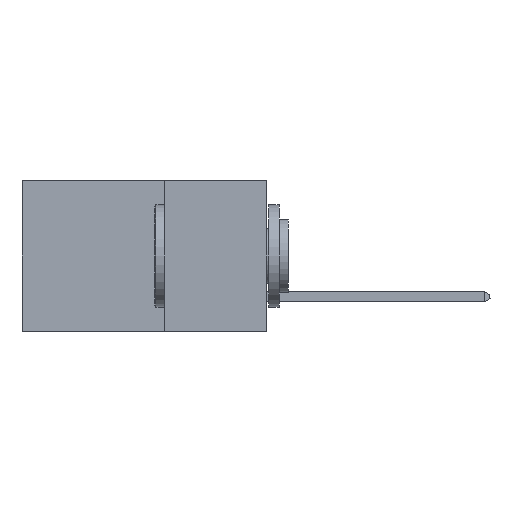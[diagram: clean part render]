
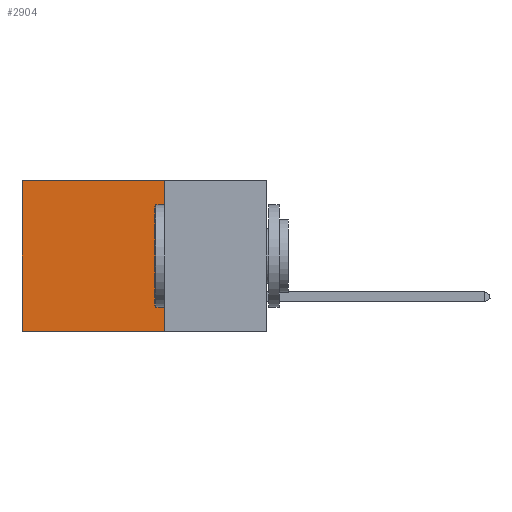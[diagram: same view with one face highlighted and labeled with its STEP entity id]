
A CAD part, left-side view. The second image highlights one B-rep face of the part: STEP entity #2904.
In plain terms, the highlighted planar face has unit normal (-1, 0, 0).
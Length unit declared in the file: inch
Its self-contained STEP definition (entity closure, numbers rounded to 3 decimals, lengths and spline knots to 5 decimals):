
#697 = CARTESIAN_POINT ( 'NONE',  ( 0.2875, 0.25, -0.37 ) ) ;
#1214 = VERTEX_POINT ( 'NONE', #697 ) ;
#2812 = DIRECTION ( 'NONE',  ( 0., 0., -1. ) ) ;
#2901 = CARTESIAN_POINT ( 'NONE',  ( 0.2875, 0.6, -0.37 ) ) ;
#2904 = ADVANCED_FACE ( 'NONE', ( #7168 ), #30668, .F. ) ;
#3519 = CARTESIAN_POINT ( 'NONE',  ( 0.2875, 0.25, 0. ) ) ;
#3806 = ORIENTED_EDGE ( 'NONE', *, *, #16122, .T. ) ;
#3827 = DIRECTION ( 'NONE',  ( 1., 0., 0. ) ) ;
#6493 = VECTOR ( 'NONE', #12857, 39.37008 ) ;
#7168 = FACE_OUTER_BOUND ( 'NONE', #11934, .T. ) ;
#8138 = ORIENTED_EDGE ( 'NONE', *, *, #24758, .F. ) ;
#8615 = VERTEX_POINT ( 'NONE', #20399 ) ;
#8788 = LINE ( 'NONE', #24919, #6493 ) ;
#8815 = VERTEX_POINT ( 'NONE', #28167 ) ;
#9678 = VERTEX_POINT ( 'NONE', #2901 ) ;
#10914 = DIRECTION ( 'NONE',  ( 0., 0., -1. ) ) ;
#11934 = EDGE_LOOP ( 'NONE', ( #28838, #25060, #8138, #3806 ) ) ;
#12069 = LINE ( 'NONE', #22989, #26578 ) ;
#12084 = EDGE_CURVE ( 'NONE', #8615, #9678, #18480, .T. ) ;
#12692 = VECTOR ( 'NONE', #2812, 39.37008 ) ;
#12857 = DIRECTION ( 'NONE',  ( 0., 1., 0. ) ) ;
#13100 = CARTESIAN_POINT ( 'NONE',  ( 0.2875, 0.25, -0.37 ) ) ;
#13912 = AXIS2_PLACEMENT_3D ( 'NONE', #3519, #3827, #10914 ) ;
#16122 = EDGE_CURVE ( 'NONE', #8815, #8615, #8788, .T. ) ;
#18480 = LINE ( 'NONE', #29619, #12692 ) ;
#20399 = CARTESIAN_POINT ( 'NONE',  ( 0.2875, 0.6, 0. ) ) ;
#20895 = EDGE_CURVE ( 'NONE', #1214, #9678, #28010, .T. ) ;
#22989 = CARTESIAN_POINT ( 'NONE',  ( 0.2875, 0.25, 0. ) ) ;
#24758 = EDGE_CURVE ( 'NONE', #8815, #1214, #12069, .T. ) ;
#24919 = CARTESIAN_POINT ( 'NONE',  ( 0.2875, 0.25, 0. ) ) ;
#25060 = ORIENTED_EDGE ( 'NONE', *, *, #20895, .F. ) ;
#25523 = DIRECTION ( 'NONE',  ( 0., 0., -1. ) ) ;
#26578 = VECTOR ( 'NONE', #25523, 39.37008 ) ;
#28010 = LINE ( 'NONE', #13100, #28772 ) ;
#28167 = CARTESIAN_POINT ( 'NONE',  ( 0.2875, 0.25, 0. ) ) ;
#28772 = VECTOR ( 'NONE', #30184, 39.37008 ) ;
#28838 = ORIENTED_EDGE ( 'NONE', *, *, #12084, .T. ) ;
#29619 = CARTESIAN_POINT ( 'NONE',  ( 0.2875, 0.6, 0. ) ) ;
#30184 = DIRECTION ( 'NONE',  ( 0., 1., 0. ) ) ;
#30668 = PLANE ( 'NONE',  #13912 ) ;
